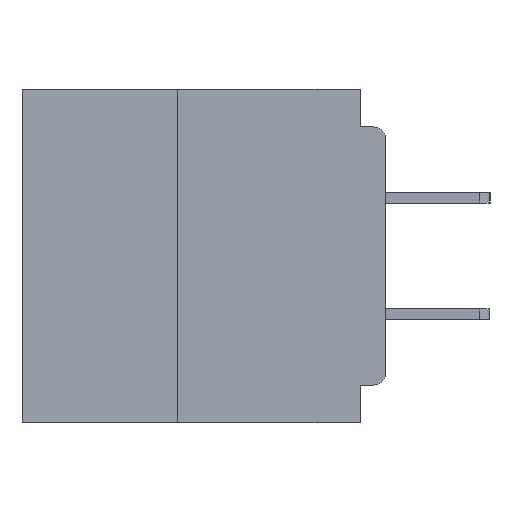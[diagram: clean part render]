
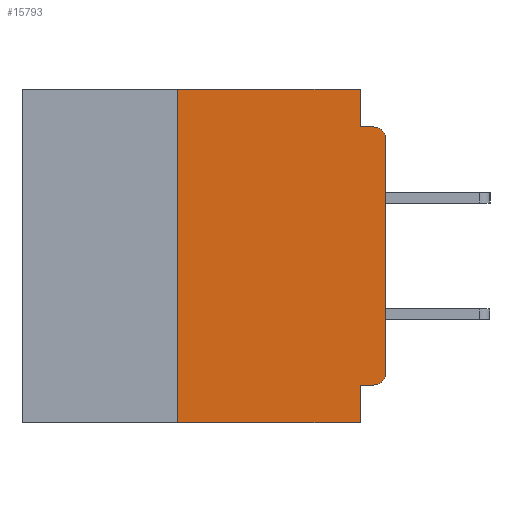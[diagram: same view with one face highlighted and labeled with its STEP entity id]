
A CAD part, left-side view. The second image highlights one B-rep face of the part: STEP entity #15793.
In plain terms, the highlighted planar face has unit normal (-1, 0, 0).
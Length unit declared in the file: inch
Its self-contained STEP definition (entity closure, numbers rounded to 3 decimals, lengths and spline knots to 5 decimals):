
#120 = VECTOR ( 'NONE', #41608, 39.37008 ) ;
#283 = DIRECTION ( 'NONE',  ( 0., 0., -1. ) ) ;
#347 = CIRCLE ( 'NONE', #36912, 0.015 ) ;
#517 = DIRECTION ( 'NONE',  ( -1., 0., 0. ) ) ;
#650 = EDGE_LOOP ( 'NONE', ( #42143, #2745, #41515, #62796, #36213, #44879, #49462, #58436, #31595, #1778 ) ) ;
#1778 = ORIENTED_EDGE ( 'NONE', *, *, #19258, .T. ) ;
#1915 = PLANE ( 'NONE',  #57899 ) ;
#2745 = ORIENTED_EDGE ( 'NONE', *, *, #18518, .T. ) ;
#2943 = VECTOR ( 'NONE', #22785, 39.37008 ) ;
#3297 = DIRECTION ( 'NONE',  ( 0., 0., 1. ) ) ;
#4654 = EDGE_CURVE ( 'NONE', #23279, #21837, #39765, .T. ) ;
#6297 = EDGE_CURVE ( 'NONE', #15184, #30550, #31674, .T. ) ;
#6331 = VECTOR ( 'NONE', #8336, 39.37008 ) ;
#6510 = DIRECTION ( 'NONE',  ( 0., 1., 0. ) ) ;
#7019 = DIRECTION ( 'NONE',  ( 0., -1., 0. ) ) ;
#8336 = DIRECTION ( 'NONE',  ( 0., 0., 1. ) ) ;
#8435 = CARTESIAN_POINT ( 'NONE',  ( 0., 0., 0. ) ) ;
#9169 = CARTESIAN_POINT ( 'NONE',  ( 0., 0.031, -0.355 ) ) ;
#10293 = EDGE_CURVE ( 'NONE', #28276, #27706, #56282, .T. ) ;
#10307 = CARTESIAN_POINT ( 'NONE',  ( 0., 0.25, 0. ) ) ;
#11804 = DIRECTION ( 'NONE',  ( 0., 0., -1. ) ) ;
#12124 = VERTEX_POINT ( 'NONE', #22714 ) ;
#12419 = EDGE_CURVE ( 'NONE', #51931, #12124, #16032, .T. ) ;
#13002 = CARTESIAN_POINT ( 'NONE',  ( 0., 0., -0.045 ) ) ;
#13195 = LINE ( 'NONE', #17125, #120 ) ;
#14587 = CARTESIAN_POINT ( 'NONE',  ( 0., 0.015, -0.06 ) ) ;
#15184 = VERTEX_POINT ( 'NONE', #17020 ) ;
#15793 = ADVANCED_FACE ( 'NONE', ( #46136 ), #1915, .F. ) ;
#16032 = LINE ( 'NONE', #13002, #2943 ) ;
#17020 = CARTESIAN_POINT ( 'NONE',  ( 0., 0.25, -0.4 ) ) ;
#17125 = CARTESIAN_POINT ( 'NONE',  ( 0., 0.031, 0. ) ) ;
#17889 = VERTEX_POINT ( 'NONE', #43102 ) ;
#18518 = EDGE_CURVE ( 'NONE', #27706, #12124, #30279, .T. ) ;
#18815 = EDGE_CURVE ( 'NONE', #32237, #17889, #49236, .T. ) ;
#19258 = EDGE_CURVE ( 'NONE', #23279, #28276, #347, .T. ) ;
#19427 = DIRECTION ( 'NONE',  ( 0., 0., -1. ) ) ;
#21035 = CARTESIAN_POINT ( 'NONE',  ( 0., 0., -0.355 ) ) ;
#21603 = EDGE_CURVE ( 'NONE', #17889, #51931, #13195, .T. ) ;
#21837 = VERTEX_POINT ( 'NONE', #9169 ) ;
#22714 = CARTESIAN_POINT ( 'NONE',  ( 0., 0.015, -0.045 ) ) ;
#22785 = DIRECTION ( 'NONE',  ( 0., -1., 0. ) ) ;
#23012 = AXIS2_PLACEMENT_3D ( 'NONE', #14587, #48602, #19427 ) ;
#23279 = VERTEX_POINT ( 'NONE', #39061 ) ;
#26825 = VECTOR ( 'NONE', #6510, 39.37008 ) ;
#27706 = VERTEX_POINT ( 'NONE', #33515 ) ;
#28276 = VERTEX_POINT ( 'NONE', #48548 ) ;
#29769 = EDGE_CURVE ( 'NONE', #21837, #30550, #43288, .T. ) ;
#29805 = CARTESIAN_POINT ( 'NONE',  ( 0., 0.015, -0.34 ) ) ;
#30279 = CIRCLE ( 'NONE', #23012, 0.015 ) ;
#30466 = VECTOR ( 'NONE', #3297, 39.37008 ) ;
#30550 = VERTEX_POINT ( 'NONE', #55382 ) ;
#31595 = ORIENTED_EDGE ( 'NONE', *, *, #4654, .F. ) ;
#31674 = LINE ( 'NONE', #49364, #43086 ) ;
#32237 = VERTEX_POINT ( 'NONE', #10307 ) ;
#33515 = CARTESIAN_POINT ( 'NONE',  ( 0., 0., -0.06 ) ) ;
#34698 = DIRECTION ( 'NONE',  ( 0., 0., -1. ) ) ;
#36100 = CARTESIAN_POINT ( 'NONE',  ( 0., 0.437, 0. ) ) ;
#36213 = ORIENTED_EDGE ( 'NONE', *, *, #18815, .F. ) ;
#36912 = AXIS2_PLACEMENT_3D ( 'NONE', #29805, #517, #34698 ) ;
#37571 = CARTESIAN_POINT ( 'NONE',  ( 0., 0.25, -0.4 ) ) ;
#39061 = CARTESIAN_POINT ( 'NONE',  ( 0., 0.015, -0.355 ) ) ;
#39765 = LINE ( 'NONE', #21035, #26825 ) ;
#40998 = DIRECTION ( 'NONE',  ( 1., 0., 0. ) ) ;
#41515 = ORIENTED_EDGE ( 'NONE', *, *, #12419, .F. ) ;
#41608 = DIRECTION ( 'NONE',  ( 0., 0., -1. ) ) ;
#41772 = VECTOR ( 'NONE', #283, 39.37008 ) ;
#42143 = ORIENTED_EDGE ( 'NONE', *, *, #10293, .T. ) ;
#43086 = VECTOR ( 'NONE', #54239, 39.37008 ) ;
#43102 = CARTESIAN_POINT ( 'NONE',  ( 0., 0.031, 0. ) ) ;
#43288 = LINE ( 'NONE', #58628, #41772 ) ;
#44879 = ORIENTED_EDGE ( 'NONE', *, *, #54733, .F. ) ;
#46034 = CARTESIAN_POINT ( 'NONE',  ( 0., 0.437, 0. ) ) ;
#46136 = FACE_OUTER_BOUND ( 'NONE', #650, .T. ) ;
#48548 = CARTESIAN_POINT ( 'NONE',  ( 0., 0., -0.34 ) ) ;
#48602 = DIRECTION ( 'NONE',  ( -1., 0., 0. ) ) ;
#49236 = LINE ( 'NONE', #46034, #62108 ) ;
#49364 = CARTESIAN_POINT ( 'NONE',  ( 0., 0.437, -0.4 ) ) ;
#49462 = ORIENTED_EDGE ( 'NONE', *, *, #6297, .T. ) ;
#51931 = VERTEX_POINT ( 'NONE', #56007 ) ;
#54239 = DIRECTION ( 'NONE',  ( 0., -1., 0. ) ) ;
#54733 = EDGE_CURVE ( 'NONE', #15184, #32237, #56610, .T. ) ;
#55382 = CARTESIAN_POINT ( 'NONE',  ( 0., 0.031, -0.4 ) ) ;
#56007 = CARTESIAN_POINT ( 'NONE',  ( 0., 0.031, -0.045 ) ) ;
#56282 = LINE ( 'NONE', #8435, #30466 ) ;
#56610 = LINE ( 'NONE', #37571, #6331 ) ;
#57899 = AXIS2_PLACEMENT_3D ( 'NONE', #36100, #40998, #11804 ) ;
#58436 = ORIENTED_EDGE ( 'NONE', *, *, #29769, .F. ) ;
#58628 = CARTESIAN_POINT ( 'NONE',  ( 0., 0.031, -0.4 ) ) ;
#62108 = VECTOR ( 'NONE', #7019, 39.37008 ) ;
#62796 = ORIENTED_EDGE ( 'NONE', *, *, #21603, .F. ) ;
